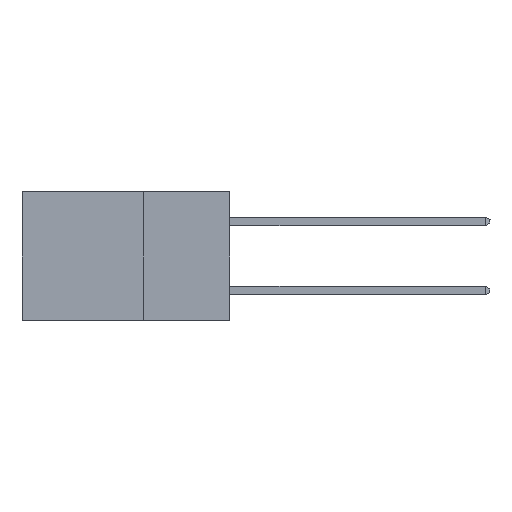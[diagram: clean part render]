
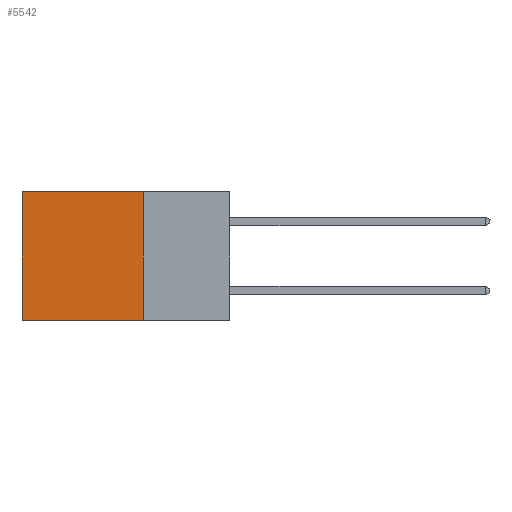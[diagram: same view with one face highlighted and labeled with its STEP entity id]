
A CAD part, left-side view. The second image highlights one B-rep face of the part: STEP entity #5542.
In plain terms, the highlighted planar face has unit normal (-1, 0, 0).
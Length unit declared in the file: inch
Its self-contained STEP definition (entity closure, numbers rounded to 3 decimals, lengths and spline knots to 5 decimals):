
#53 = EDGE_CURVE ( 'NONE', #6233, #3002, #4756, .T. ) ;
#649 = VERTEX_POINT ( 'NONE', #13301 ) ;
#1677 = VECTOR ( 'NONE', #5143, 39.37008 ) ;
#2217 = DIRECTION ( 'NONE',  ( 1., 0., 0. ) ) ;
#2639 = DIRECTION ( 'NONE',  ( 0., 1., 0. ) ) ;
#2988 = EDGE_CURVE ( 'NONE', #3002, #649, #5107, .T. ) ;
#2993 = AXIS2_PLACEMENT_3D ( 'NONE', #11582, #2217, #10535 ) ;
#3002 = VERTEX_POINT ( 'NONE', #4208 ) ;
#3851 = ORIENTED_EDGE ( 'NONE', *, *, #8936, .F. ) ;
#4191 = CARTESIAN_POINT ( 'NONE',  ( 0.2615, 0.25, -0.37 ) ) ;
#4208 = CARTESIAN_POINT ( 'NONE',  ( 0.2615, 0.6, 0. ) ) ;
#4756 = LINE ( 'NONE', #6953, #7392 ) ;
#5107 = LINE ( 'NONE', #10564, #6123 ) ;
#5143 = DIRECTION ( 'NONE',  ( 0., 0., -1. ) ) ;
#5238 = VERTEX_POINT ( 'NONE', #4191 ) ;
#5253 = DIRECTION ( 'NONE',  ( 0., 0., -1. ) ) ;
#5268 = ORIENTED_EDGE ( 'NONE', *, *, #10947, .F. ) ;
#5542 = ADVANCED_FACE ( 'NONE', ( #12590 ), #7407, .F. ) ;
#5881 = CARTESIAN_POINT ( 'NONE',  ( 0.2615, 0.25, 0. ) ) ;
#5997 = DIRECTION ( 'NONE',  ( 0., 1., 0. ) ) ;
#6083 = ORIENTED_EDGE ( 'NONE', *, *, #53, .T. ) ;
#6123 = VECTOR ( 'NONE', #5253, 39.37008 ) ;
#6233 = VERTEX_POINT ( 'NONE', #5881 ) ;
#6953 = CARTESIAN_POINT ( 'NONE',  ( 0.2615, 0.25, 0. ) ) ;
#7309 = VECTOR ( 'NONE', #2639, 39.37008 ) ;
#7392 = VECTOR ( 'NONE', #5997, 39.37008 ) ;
#7407 = PLANE ( 'NONE',  #2993 ) ;
#8936 = EDGE_CURVE ( 'NONE', #5238, #649, #11997, .T. ) ;
#10065 = EDGE_LOOP ( 'NONE', ( #12112, #3851, #5268, #6083 ) ) ;
#10313 = CARTESIAN_POINT ( 'NONE',  ( 0.2615, 0.25, -0.37 ) ) ;
#10535 = DIRECTION ( 'NONE',  ( 0., 0., -1. ) ) ;
#10564 = CARTESIAN_POINT ( 'NONE',  ( 0.2615, 0.6, -0.37 ) ) ;
#10947 = EDGE_CURVE ( 'NONE', #6233, #5238, #12458, .T. ) ;
#10971 = CARTESIAN_POINT ( 'NONE',  ( 0.2615, 0.25, -0.37 ) ) ;
#11582 = CARTESIAN_POINT ( 'NONE',  ( 0.2615, 0.25, -0.37 ) ) ;
#11997 = LINE ( 'NONE', #10971, #7309 ) ;
#12112 = ORIENTED_EDGE ( 'NONE', *, *, #2988, .T. ) ;
#12458 = LINE ( 'NONE', #10313, #1677 ) ;
#12590 = FACE_OUTER_BOUND ( 'NONE', #10065, .T. ) ;
#13301 = CARTESIAN_POINT ( 'NONE',  ( 0.2615, 0.6, -0.37 ) ) ;
